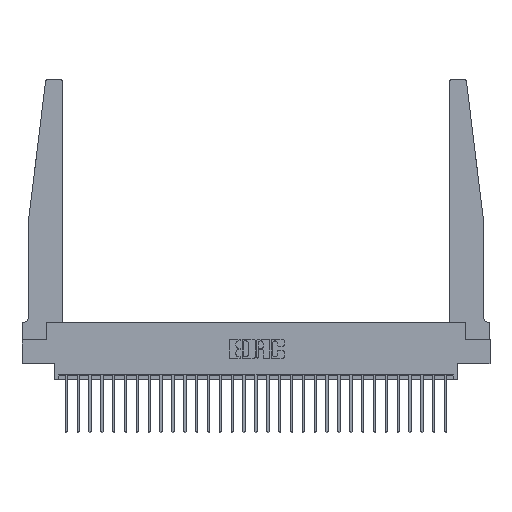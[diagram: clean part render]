
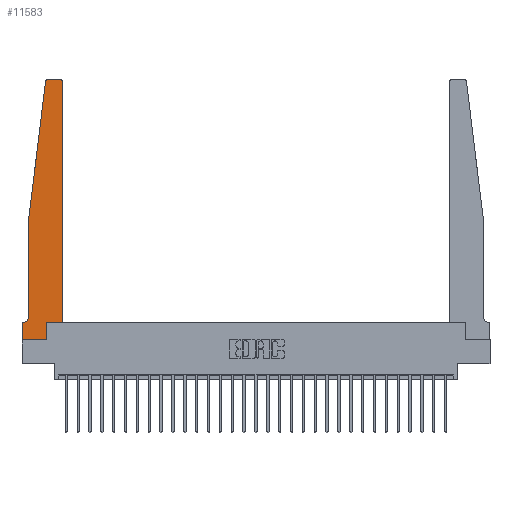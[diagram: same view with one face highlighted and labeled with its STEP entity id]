
A CAD part, top view. The second image highlights one B-rep face of the part: STEP entity #11583.
In plain terms, the highlighted planar face has unit normal (0, 0, 1).
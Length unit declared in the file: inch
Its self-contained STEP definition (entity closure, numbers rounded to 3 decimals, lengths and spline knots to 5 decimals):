
#690 = ORIENTED_EDGE ( 'NONE', *, *, #11139, .T. ) ;
#827 = VECTOR ( 'NONE', #5056, 39.37008 ) ;
#1046 = DIRECTION ( 'NONE',  ( 1., 0., 0. ) ) ;
#1101 = DIRECTION ( 'NONE',  ( 0., -1., 0. ) ) ;
#1499 = EDGE_CURVE ( 'NONE', #4011, #13898, #26323, .T. ) ;
#1721 = CARTESIAN_POINT ( 'NONE',  ( 0.2605, 0., 0.37 ) ) ;
#1862 = ORIENTED_EDGE ( 'NONE', *, *, #11912, .T. ) ;
#1913 = EDGE_CURVE ( 'NONE', #24079, #17713, #20178, .T. ) ;
#2541 = ORIENTED_EDGE ( 'NONE', *, *, #1499, .T. ) ;
#2814 = CARTESIAN_POINT ( 'NONE',  ( 0.015, 0.2375, 0.37 ) ) ;
#3189 = CARTESIAN_POINT ( 'NONE',  ( 0.425, 0.18, 0.37 ) ) ;
#3533 = AXIS2_PLACEMENT_3D ( 'NONE', #2814, #16086, #24605 ) ;
#3559 = CARTESIAN_POINT ( 'NONE',  ( 0.065, 1.25, 0.37 ) ) ;
#3857 = ORIENTED_EDGE ( 'NONE', *, *, #21759, .T. ) ;
#3870 = EDGE_CURVE ( 'NONE', #20913, #4011, #24401, .T. ) ;
#4011 = VERTEX_POINT ( 'NONE', #5482 ) ;
#4519 = DIRECTION ( 'NONE',  ( -1., 0., 0. ) ) ;
#4598 = EDGE_CURVE ( 'NONE', #24121, #9263, #7374, .T. ) ;
#5056 = DIRECTION ( 'NONE',  ( 0., 1., 0. ) ) ;
#5236 = DIRECTION ( 'NONE',  ( 0., 0., 1. ) ) ;
#5482 = CARTESIAN_POINT ( 'NONE',  ( 0., 0., 0.37 ) ) ;
#5926 = CARTESIAN_POINT ( 'NONE',  ( 0.065, 1.25, 0.37 ) ) ;
#6691 = DIRECTION ( 'NONE',  ( 1., 0., 0. ) ) ;
#6758 = AXIS2_PLACEMENT_3D ( 'NONE', #20218, #5236, #24739 ) ;
#6816 = CIRCLE ( 'NONE', #19075, 0.03 ) ;
#7123 = CARTESIAN_POINT ( 'NONE',  ( 0.065, 1.25, 0.37 ) ) ;
#7185 = CARTESIAN_POINT ( 'NONE',  ( 0.425, 0.18, 0.37 ) ) ;
#7306 = DIRECTION ( 'NONE',  ( 0., 1., 0. ) ) ;
#7374 = LINE ( 'NONE', #24973, #13805 ) ;
#7506 = EDGE_LOOP ( 'NONE', ( #1862, #21810, #3857, #9462, #12873, #17882, #13993, #2541, #690, #14241, #24663, #7702 ) ) ;
#7637 = EDGE_CURVE ( 'NONE', #24400, #23498, #6816, .T. ) ;
#7702 = ORIENTED_EDGE ( 'NONE', *, *, #7637, .T. ) ;
#8438 = CARTESIAN_POINT ( 'NONE',  ( 0., 0., 0.37 ) ) ;
#8741 = LINE ( 'NONE', #18104, #21817 ) ;
#9263 = VERTEX_POINT ( 'NONE', #7185 ) ;
#9462 = ORIENTED_EDGE ( 'NONE', *, *, #11567, .T. ) ;
#9927 = VECTOR ( 'NONE', #27265, 39.37008 ) ;
#10664 = CARTESIAN_POINT ( 'NONE',  ( 0.065, 0.1875, 0.37 ) ) ;
#10934 = DIRECTION ( 'NONE',  ( -1., 0., 0. ) ) ;
#11139 = EDGE_CURVE ( 'NONE', #13898, #24121, #8741, .T. ) ;
#11526 = DIRECTION ( 'NONE',  ( 0., 0., 1. ) ) ;
#11533 = EDGE_CURVE ( 'NONE', #18139, #27052, #15868, .T. ) ;
#11542 = VECTOR ( 'NONE', #24128, 39.37008 ) ;
#11567 = EDGE_CURVE ( 'NONE', #13626, #18139, #15960, .T. ) ;
#11583 = ADVANCED_FACE ( 'NONE', ( #20757 ), #15805, .T. ) ;
#11614 = LINE ( 'NONE', #3189, #827 ) ;
#11912 = EDGE_CURVE ( 'NONE', #23498, #24079, #19465, .T. ) ;
#12713 = VECTOR ( 'NONE', #6691, 39.37008 ) ;
#12873 = ORIENTED_EDGE ( 'NONE', *, *, #11533, .T. ) ;
#13626 = VERTEX_POINT ( 'NONE', #3559 ) ;
#13805 = VECTOR ( 'NONE', #24690, 39.37008 ) ;
#13898 = VERTEX_POINT ( 'NONE', #1721 ) ;
#13993 = ORIENTED_EDGE ( 'NONE', *, *, #3870, .T. ) ;
#14026 = CARTESIAN_POINT ( 'NONE',  ( 0.395, 2.72, 0.37 ) ) ;
#14241 = ORIENTED_EDGE ( 'NONE', *, *, #4598, .T. ) ;
#14522 = VECTOR ( 'NONE', #10934, 39.37008 ) ;
#14978 = VECTOR ( 'NONE', #1101, 39.37008 ) ;
#15780 = CARTESIAN_POINT ( 'NONE',  ( 0.065, 0.2375, 0.37 ) ) ;
#15805 = PLANE ( 'NONE',  #6758 ) ;
#15813 = CARTESIAN_POINT ( 'NONE',  ( 0.24675, 2.72367, 0.37 ) ) ;
#15849 = CARTESIAN_POINT ( 'NONE',  ( 0.015, 0.1875, 0.37 ) ) ;
#15868 = CIRCLE ( 'NONE', #3533, 0.05 ) ;
#15960 = LINE ( 'NONE', #7123, #14978 ) ;
#16086 = DIRECTION ( 'NONE',  ( 0., 0., -1. ) ) ;
#16971 = CARTESIAN_POINT ( 'NONE',  ( 0.27653, 2.75, 0.37 ) ) ;
#17472 = CARTESIAN_POINT ( 'NONE',  ( 0.25, 2.75, 0.37 ) ) ;
#17713 = VERTEX_POINT ( 'NONE', #15813 ) ;
#17882 = ORIENTED_EDGE ( 'NONE', *, *, #21383, .T. ) ;
#18104 = CARTESIAN_POINT ( 'NONE',  ( 0.2605, 0.18, 0.37 ) ) ;
#18139 = VERTEX_POINT ( 'NONE', #15780 ) ;
#19075 = AXIS2_PLACEMENT_3D ( 'NONE', #14026, #20579, #1046 ) ;
#19465 = LINE ( 'NONE', #17472, #14522 ) ;
#20178 = CIRCLE ( 'NONE', #21965, 0.03 ) ;
#20218 = CARTESIAN_POINT ( 'NONE',  ( 0., 0.1875, 0.37 ) ) ;
#20297 = CARTESIAN_POINT ( 'NONE',  ( 0., 0., 0.37 ) ) ;
#20579 = DIRECTION ( 'NONE',  ( 0., 0., 1. ) ) ;
#20757 = FACE_OUTER_BOUND ( 'NONE', #7506, .T. ) ;
#20913 = VERTEX_POINT ( 'NONE', #23896 ) ;
#21383 = EDGE_CURVE ( 'NONE', #27052, #20913, #21615, .T. ) ;
#21615 = LINE ( 'NONE', #10664, #23515 ) ;
#21759 = EDGE_CURVE ( 'NONE', #17713, #13626, #22988, .T. ) ;
#21810 = ORIENTED_EDGE ( 'NONE', *, *, #1913, .T. ) ;
#21817 = VECTOR ( 'NONE', #7306, 39.37008 ) ;
#21965 = AXIS2_PLACEMENT_3D ( 'NONE', #22335, #11526, #22179 ) ;
#22179 = DIRECTION ( 'NONE',  ( 1., 0., 0. ) ) ;
#22335 = CARTESIAN_POINT ( 'NONE',  ( 0.27653, 2.72, 0.37 ) ) ;
#22966 = CARTESIAN_POINT ( 'NONE',  ( 0.395, 2.75, 0.37 ) ) ;
#22988 = LINE ( 'NONE', #5926, #9927 ) ;
#23348 = EDGE_CURVE ( 'NONE', #9263, #24400, #11614, .T. ) ;
#23452 = CARTESIAN_POINT ( 'NONE',  ( 0.425, 2.72, 0.37 ) ) ;
#23498 = VERTEX_POINT ( 'NONE', #22966 ) ;
#23515 = VECTOR ( 'NONE', #4519, 39.37008 ) ;
#23896 = CARTESIAN_POINT ( 'NONE',  ( 0., 0.1875, 0.37 ) ) ;
#24079 = VERTEX_POINT ( 'NONE', #16971 ) ;
#24121 = VERTEX_POINT ( 'NONE', #26055 ) ;
#24128 = DIRECTION ( 'NONE',  ( 0., -1., 0. ) ) ;
#24400 = VERTEX_POINT ( 'NONE', #23452 ) ;
#24401 = LINE ( 'NONE', #20297, #11542 ) ;
#24605 = DIRECTION ( 'NONE',  ( -1., 0., 0. ) ) ;
#24663 = ORIENTED_EDGE ( 'NONE', *, *, #23348, .T. ) ;
#24690 = DIRECTION ( 'NONE',  ( 1., 0., 0. ) ) ;
#24739 = DIRECTION ( 'NONE',  ( 1., 0., 0. ) ) ;
#24973 = CARTESIAN_POINT ( 'NONE',  ( 0.425, 0.18, 0.37 ) ) ;
#26055 = CARTESIAN_POINT ( 'NONE',  ( 0.2605, 0.18, 0.37 ) ) ;
#26323 = LINE ( 'NONE', #8438, #12713 ) ;
#27052 = VERTEX_POINT ( 'NONE', #15849 ) ;
#27265 = DIRECTION ( 'NONE',  ( -0.122, -0.992, 0. ) ) ;
